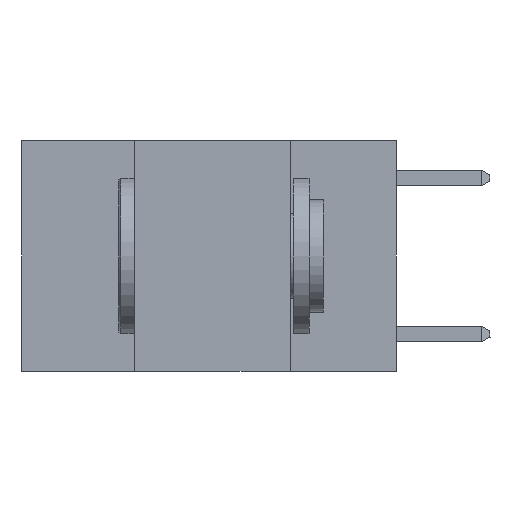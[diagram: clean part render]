
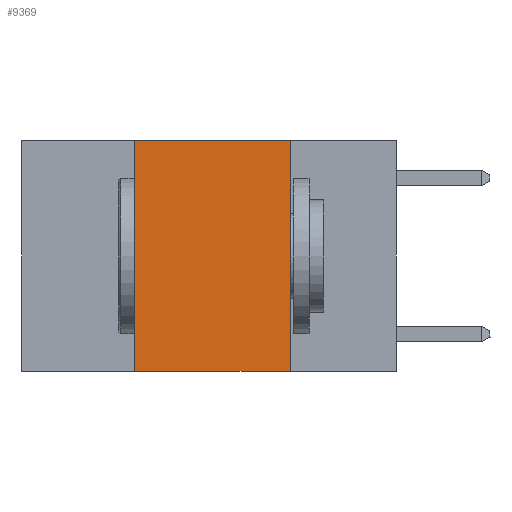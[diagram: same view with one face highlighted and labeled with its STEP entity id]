
A CAD part, left-side view. The second image highlights one B-rep face of the part: STEP entity #9369.
In plain terms, the highlighted planar face has unit normal (-1, 0, 0).
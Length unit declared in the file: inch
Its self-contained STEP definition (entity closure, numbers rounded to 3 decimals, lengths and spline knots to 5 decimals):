
#324 = VERTEX_POINT ( 'NONE', #16638 ) ;
#484 = DIRECTION ( 'NONE',  ( 0., 0., -1. ) ) ;
#1516 = VECTOR ( 'NONE', #11974, 39.37008 ) ;
#2145 = CARTESIAN_POINT ( 'NONE',  ( 0., 0.17, -0.37 ) ) ;
#2251 = EDGE_CURVE ( 'NONE', #9543, #7553, #10629, .T. ) ;
#2618 = ORIENTED_EDGE ( 'NONE', *, *, #10766, .F. ) ;
#3038 = CARTESIAN_POINT ( 'NONE',  ( 0., 0.42, 0. ) ) ;
#3450 = VECTOR ( 'NONE', #4805, 39.37008 ) ;
#4805 = DIRECTION ( 'NONE',  ( 0., 0., 1. ) ) ;
#5245 = EDGE_CURVE ( 'NONE', #11004, #7553, #9432, .T. ) ;
#6248 = FACE_OUTER_BOUND ( 'NONE', #12367, .T. ) ;
#6526 = VECTOR ( 'NONE', #8509, 39.37008 ) ;
#7011 = ORIENTED_EDGE ( 'NONE', *, *, #5245, .F. ) ;
#7553 = VERTEX_POINT ( 'NONE', #2145 ) ;
#7936 = PLANE ( 'NONE',  #9823 ) ;
#8331 = CARTESIAN_POINT ( 'NONE',  ( 0., 0.42, -0.37 ) ) ;
#8509 = DIRECTION ( 'NONE',  ( 0., -1., 0. ) ) ;
#8563 = DIRECTION ( 'NONE',  ( 0., -1., 0. ) ) ;
#8646 = EDGE_CURVE ( 'NONE', #324, #11004, #18019, .T. ) ;
#9369 = ADVANCED_FACE ( 'NONE', ( #6248 ), #7936, .F. ) ;
#9402 = CARTESIAN_POINT ( 'NONE',  ( 0., 0.6, 0. ) ) ;
#9432 = LINE ( 'NONE', #14900, #1516 ) ;
#9462 = DIRECTION ( 'NONE',  ( 1., 0., 0. ) ) ;
#9543 = VERTEX_POINT ( 'NONE', #8331 ) ;
#9823 = AXIS2_PLACEMENT_3D ( 'NONE', #9402, #9462, #484 ) ;
#10629 = LINE ( 'NONE', #18568, #14947 ) ;
#10766 = EDGE_CURVE ( 'NONE', #9543, #324, #15117, .T. ) ;
#10903 = ORIENTED_EDGE ( 'NONE', *, *, #8646, .F. ) ;
#11004 = VERTEX_POINT ( 'NONE', #18295 ) ;
#11974 = DIRECTION ( 'NONE',  ( 0., 0., -1. ) ) ;
#12306 = ORIENTED_EDGE ( 'NONE', *, *, #2251, .T. ) ;
#12367 = EDGE_LOOP ( 'NONE', ( #7011, #10903, #2618, #12306 ) ) ;
#14900 = CARTESIAN_POINT ( 'NONE',  ( 0., 0.17, 0. ) ) ;
#14947 = VECTOR ( 'NONE', #8563, 39.37008 ) ;
#15117 = LINE ( 'NONE', #3038, #3450 ) ;
#15720 = CARTESIAN_POINT ( 'NONE',  ( 0., 0.6, 0. ) ) ;
#16638 = CARTESIAN_POINT ( 'NONE',  ( 0., 0.42, 0. ) ) ;
#18019 = LINE ( 'NONE', #15720, #6526 ) ;
#18295 = CARTESIAN_POINT ( 'NONE',  ( 0., 0.17, 0. ) ) ;
#18568 = CARTESIAN_POINT ( 'NONE',  ( 0., 0.6, -0.37 ) ) ;
